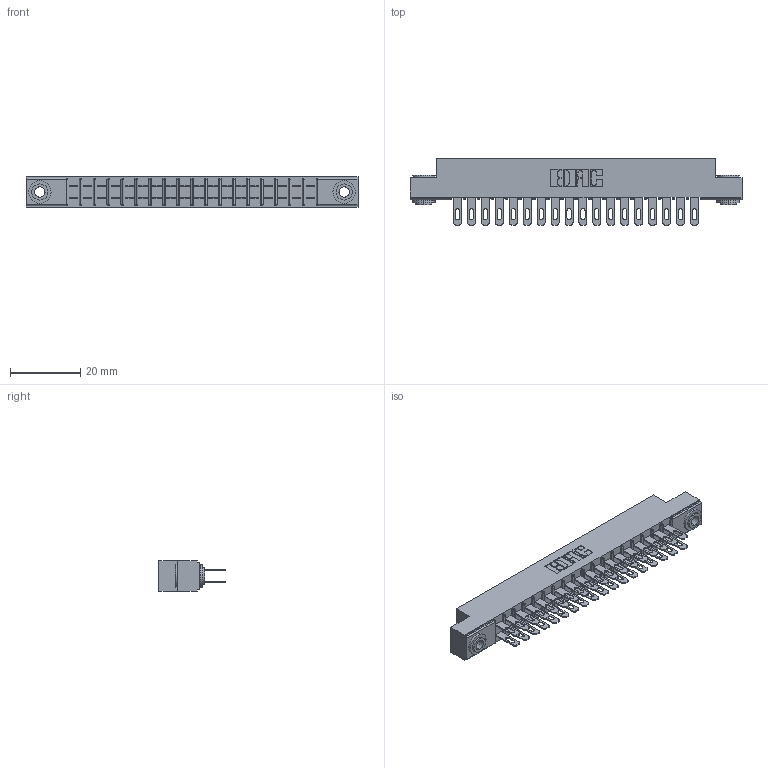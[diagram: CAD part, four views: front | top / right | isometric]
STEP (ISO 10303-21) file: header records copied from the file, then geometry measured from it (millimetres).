
FILE_DESCRIPTION (( 'STEP AP203' ), '1' );
FILE_NAME ('355-036-500-203.STEP', '2019-09-11T09:15:28', ( '' ), ( '' ), 'SwSTEP 2.0', 'SolidWorks 2016', '' );
FILE_SCHEMA (( 'CONFIG_CONTROL_DESIGN' ));
Length unit declared in the file: inch
Products named in the file (4): 355-036-500-203; 305 Part_.156 Dia; 305-290-001_500; 345-250-002_345-250-002-102
Assembly tree (39 placements, depth 2):
  355-036-500-203
    305 Part_.156 Dia
    305-290-001_500  x36
    345-250-002_345-250-002-102  x2
Bounding box: 94.34 x 18.85 x 8.71 mm (x, y, z)
Volume: 6031 mm3; surface area: 12046.3 mm2
Topology: 39 solids, 39 shells, 1968 faces, 5594 edges, 3628 vertices
Faces by surface type: plane 1100, cylinder 788, sphere 72, cone 8
Entity records: 23498 total; most frequent: CARTESIAN_POINT 3869, ORIENTED_EDGE 3828, DIRECTION 3780, EDGE_CURVE 1914, LINE 1510, VECTOR 1510, VERTEX_POINT 1224, AXIS2_PLACEMENT_3D 1135
